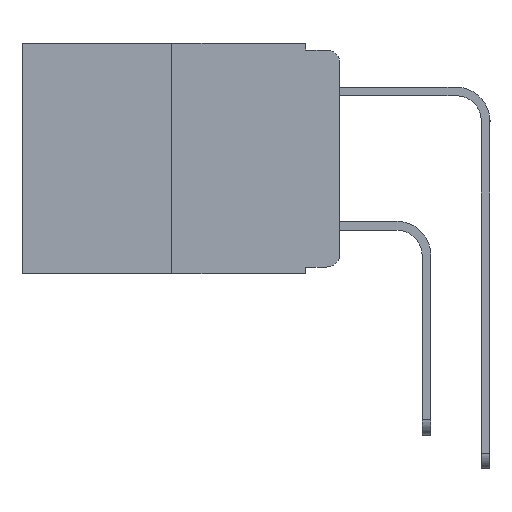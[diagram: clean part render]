
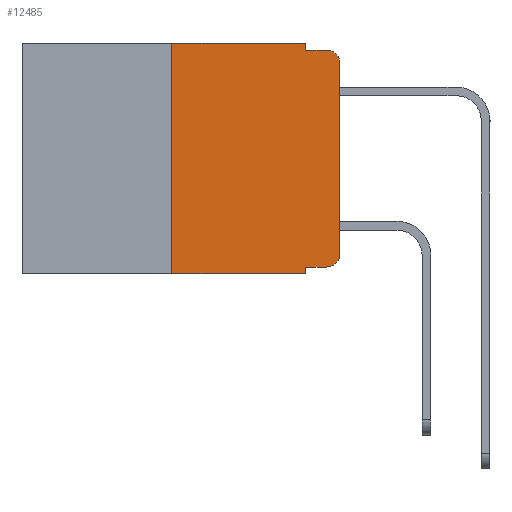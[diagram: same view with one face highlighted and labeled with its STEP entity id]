
A CAD part, left-side view. The second image highlights one B-rep face of the part: STEP entity #12485.
In plain terms, the highlighted planar face has unit normal (-1, 0, 0).
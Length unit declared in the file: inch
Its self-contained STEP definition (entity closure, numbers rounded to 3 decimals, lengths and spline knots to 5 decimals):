
#137 = ORIENTED_EDGE ( 'NONE', *, *, #7662, .F. ) ;
#380 = CARTESIAN_POINT ( 'NONE',  ( 0., 0., 0. ) ) ;
#817 = VECTOR ( 'NONE', #11443, 39.37008 ) ;
#844 = PLANE ( 'NONE',  #5195 ) ;
#865 = DIRECTION ( 'NONE',  ( -1., 0., 0. ) ) ;
#1127 = CARTESIAN_POINT ( 'NONE',  ( 0., 0., -0.03 ) ) ;
#1220 = LINE ( 'NONE', #10141, #7373 ) ;
#1554 = AXIS2_PLACEMENT_3D ( 'NONE', #11621, #5204, #12698 ) ;
#1746 = FACE_OUTER_BOUND ( 'NONE', #12675, .T. ) ;
#1765 = ORIENTED_EDGE ( 'NONE', *, *, #12231, .F. ) ;
#1789 = VERTEX_POINT ( 'NONE', #3589 ) ;
#1797 = CARTESIAN_POINT ( 'NONE',  ( 0., 0.02, -0.01 ) ) ;
#1846 = VECTOR ( 'NONE', #10717, 39.37008 ) ;
#1859 = CARTESIAN_POINT ( 'NONE',  ( 0., 0.051, -0.333 ) ) ;
#1918 = VERTEX_POINT ( 'NONE', #3889 ) ;
#1958 = LINE ( 'NONE', #6520, #7798 ) ;
#2172 = DIRECTION ( 'NONE',  ( 1., 0., 0. ) ) ;
#3314 = LINE ( 'NONE', #12382, #5672 ) ;
#3352 = ORIENTED_EDGE ( 'NONE', *, *, #5757, .T. ) ;
#3386 = ORIENTED_EDGE ( 'NONE', *, *, #8367, .T. ) ;
#3556 = ORIENTED_EDGE ( 'NONE', *, *, #4858, .F. ) ;
#3589 = CARTESIAN_POINT ( 'NONE',  ( 0., 0., -0.313 ) ) ;
#3889 = CARTESIAN_POINT ( 'NONE',  ( 0., 0.25, 0. ) ) ;
#4192 = LINE ( 'NONE', #7213, #817 ) ;
#4317 = ORIENTED_EDGE ( 'NONE', *, *, #6129, .T. ) ;
#4374 = VERTEX_POINT ( 'NONE', #8344 ) ;
#4416 = LINE ( 'NONE', #7006, #7077 ) ;
#4683 = ORIENTED_EDGE ( 'NONE', *, *, #13512, .F. ) ;
#4858 = EDGE_CURVE ( 'NONE', #12117, #13857, #4192, .T. ) ;
#4939 = EDGE_CURVE ( 'NONE', #10038, #13857, #11817, .T. ) ;
#5195 = AXIS2_PLACEMENT_3D ( 'NONE', #5720, #2172, #10043 ) ;
#5204 = DIRECTION ( 'NONE',  ( -1., 0., 0. ) ) ;
#5256 = EDGE_CURVE ( 'NONE', #6511, #6213, #1220, .T. ) ;
#5636 = AXIS2_PLACEMENT_3D ( 'NONE', #7958, #865, #9001 ) ;
#5672 = VECTOR ( 'NONE', #5994, 39.37008 ) ;
#5720 = CARTESIAN_POINT ( 'NONE',  ( 0., 0.473, 0. ) ) ;
#5757 = EDGE_CURVE ( 'NONE', #1789, #10038, #11161, .T. ) ;
#5994 = DIRECTION ( 'NONE',  ( 0., 0., -1. ) ) ;
#6129 = EDGE_CURVE ( 'NONE', #14036, #11554, #9979, .T. ) ;
#6213 = VERTEX_POINT ( 'NONE', #8417 ) ;
#6391 = LINE ( 'NONE', #11352, #8903 ) ;
#6511 = VERTEX_POINT ( 'NONE', #1859 ) ;
#6520 = CARTESIAN_POINT ( 'NONE',  ( 0., 0.051, 0. ) ) ;
#6594 = CARTESIAN_POINT ( 'NONE',  ( 0., 0.051, -0.343 ) ) ;
#7006 = CARTESIAN_POINT ( 'NONE',  ( 0., 0.473, 0. ) ) ;
#7077 = VECTOR ( 'NONE', #13334, 39.37008 ) ;
#7213 = CARTESIAN_POINT ( 'NONE',  ( 0., 0.051, -0.01 ) ) ;
#7373 = VECTOR ( 'NONE', #13353, 39.37008 ) ;
#7662 = EDGE_CURVE ( 'NONE', #1918, #4374, #4416, .T. ) ;
#7798 = VECTOR ( 'NONE', #9668, 39.37008 ) ;
#7958 = CARTESIAN_POINT ( 'NONE',  ( 0., 0.02, -0.313 ) ) ;
#8281 = CARTESIAN_POINT ( 'NONE',  ( 0., 0.473, -0.343 ) ) ;
#8344 = CARTESIAN_POINT ( 'NONE',  ( 0., 0.051, 0. ) ) ;
#8367 = EDGE_CURVE ( 'NONE', #6213, #1789, #10999, .T. ) ;
#8417 = CARTESIAN_POINT ( 'NONE',  ( 0., 0.02, -0.333 ) ) ;
#8903 = VECTOR ( 'NONE', #12415, 39.37008 ) ;
#9001 = DIRECTION ( 'NONE',  ( 0., 0., -1. ) ) ;
#9315 = DIRECTION ( 'NONE',  ( 0., -1., 0. ) ) ;
#9424 = ORIENTED_EDGE ( 'NONE', *, *, #14290, .F. ) ;
#9576 = ORIENTED_EDGE ( 'NONE', *, *, #4939, .T. ) ;
#9642 = VECTOR ( 'NONE', #9315, 39.37008 ) ;
#9668 = DIRECTION ( 'NONE',  ( 0., 0., -1. ) ) ;
#9979 = LINE ( 'NONE', #8281, #9642 ) ;
#10038 = VERTEX_POINT ( 'NONE', #1127 ) ;
#10043 = DIRECTION ( 'NONE',  ( 0., 0., -1. ) ) ;
#10141 = CARTESIAN_POINT ( 'NONE',  ( 0., 0.051, -0.333 ) ) ;
#10717 = DIRECTION ( 'NONE',  ( 0., 0., 1. ) ) ;
#10764 = ORIENTED_EDGE ( 'NONE', *, *, #5256, .T. ) ;
#10999 = CIRCLE ( 'NONE', #5636, 0.02 ) ;
#11161 = LINE ( 'NONE', #380, #1846 ) ;
#11352 = CARTESIAN_POINT ( 'NONE',  ( 0., 0.25, 0. ) ) ;
#11443 = DIRECTION ( 'NONE',  ( 0., -1., 0. ) ) ;
#11478 = CARTESIAN_POINT ( 'NONE',  ( 0., 0.051, -0.01 ) ) ;
#11554 = VERTEX_POINT ( 'NONE', #6594 ) ;
#11621 = CARTESIAN_POINT ( 'NONE',  ( 0., 0.02, -0.03 ) ) ;
#11817 = CIRCLE ( 'NONE', #1554, 0.02 ) ;
#12044 = CARTESIAN_POINT ( 'NONE',  ( 0., 0.25, -0.343 ) ) ;
#12117 = VERTEX_POINT ( 'NONE', #11478 ) ;
#12231 = EDGE_CURVE ( 'NONE', #4374, #12117, #1958, .T. ) ;
#12382 = CARTESIAN_POINT ( 'NONE',  ( 0., 0.051, 0. ) ) ;
#12415 = DIRECTION ( 'NONE',  ( 0., 0., 1. ) ) ;
#12485 = ADVANCED_FACE ( 'NONE', ( #1746 ), #844, .F. ) ;
#12675 = EDGE_LOOP ( 'NONE', ( #3352, #9576, #3556, #1765, #137, #9424, #4317, #4683, #10764, #3386 ) ) ;
#12698 = DIRECTION ( 'NONE',  ( 0., 0., -1. ) ) ;
#13334 = DIRECTION ( 'NONE',  ( 0., -1., 0. ) ) ;
#13353 = DIRECTION ( 'NONE',  ( 0., -1., 0. ) ) ;
#13512 = EDGE_CURVE ( 'NONE', #6511, #11554, #3314, .T. ) ;
#13857 = VERTEX_POINT ( 'NONE', #1797 ) ;
#14036 = VERTEX_POINT ( 'NONE', #12044 ) ;
#14290 = EDGE_CURVE ( 'NONE', #14036, #1918, #6391, .T. ) ;
